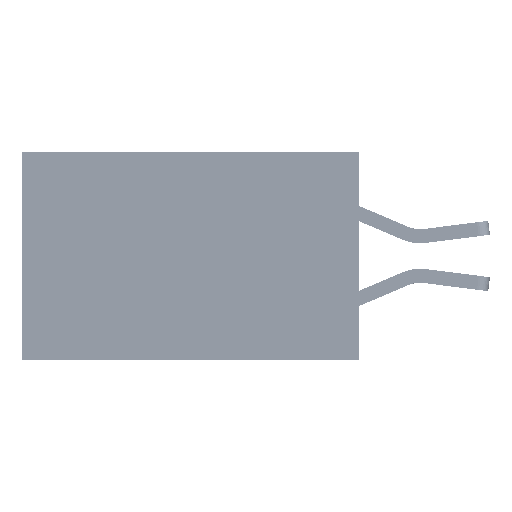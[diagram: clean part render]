
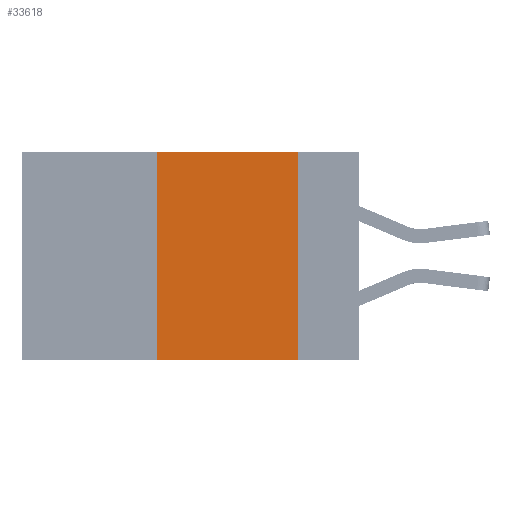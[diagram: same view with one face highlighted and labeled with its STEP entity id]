
A CAD part, left-side view. The second image highlights one B-rep face of the part: STEP entity #33618.
In plain terms, the highlighted planar face has unit normal (-1, 0, 0).
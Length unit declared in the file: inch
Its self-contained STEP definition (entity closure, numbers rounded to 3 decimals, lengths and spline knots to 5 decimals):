
#204 = LINE ( 'NONE', #19303, #33408 ) ;
#1586 = VERTEX_POINT ( 'NONE', #36401 ) ;
#2526 = VECTOR ( 'NONE', #12789, 39.37008 ) ;
#2970 = EDGE_CURVE ( 'NONE', #21396, #1586, #34443, .T. ) ;
#3030 = CARTESIAN_POINT ( 'NONE',  ( 0., 0.11, -0.37 ) ) ;
#3728 = EDGE_CURVE ( 'NONE', #21396, #26308, #35693, .T. ) ;
#4041 = ORIENTED_EDGE ( 'NONE', *, *, #3728, .T. ) ;
#4590 = LINE ( 'NONE', #7376, #32959 ) ;
#6262 = ORIENTED_EDGE ( 'NONE', *, *, #6653, .F. ) ;
#6653 = EDGE_CURVE ( 'NONE', #1586, #18485, #4590, .T. ) ;
#7141 = DIRECTION ( 'NONE',  ( 0., -1., 0. ) ) ;
#7376 = CARTESIAN_POINT ( 'NONE',  ( 0., 0.6, 0. ) ) ;
#11232 = FACE_OUTER_BOUND ( 'NONE', #19173, .T. ) ;
#11411 = PLANE ( 'NONE',  #26096 ) ;
#12393 = DIRECTION ( 'NONE',  ( 1., 0., 0. ) ) ;
#12789 = DIRECTION ( 'NONE',  ( 0., 0., 1. ) ) ;
#17364 = CARTESIAN_POINT ( 'NONE',  ( 0., 0.6, 0. ) ) ;
#17844 = DIRECTION ( 'NONE',  ( 0., 0., -1. ) ) ;
#18485 = VERTEX_POINT ( 'NONE', #23875 ) ;
#19173 = EDGE_LOOP ( 'NONE', ( #26755, #6262, #34227, #4041 ) ) ;
#19303 = CARTESIAN_POINT ( 'NONE',  ( 0., 0.11, 0. ) ) ;
#19483 = CARTESIAN_POINT ( 'NONE',  ( 0., 0.36, -0.37 ) ) ;
#21166 = CARTESIAN_POINT ( 'NONE',  ( 0., 0.6, -0.37 ) ) ;
#21396 = VERTEX_POINT ( 'NONE', #19483 ) ;
#23734 = EDGE_CURVE ( 'NONE', #18485, #26308, #204, .T. ) ;
#23875 = CARTESIAN_POINT ( 'NONE',  ( 0., 0.11, 0. ) ) ;
#26096 = AXIS2_PLACEMENT_3D ( 'NONE', #17364, #12393, #17844 ) ;
#26308 = VERTEX_POINT ( 'NONE', #3030 ) ;
#26755 = ORIENTED_EDGE ( 'NONE', *, *, #23734, .F. ) ;
#26996 = DIRECTION ( 'NONE',  ( 0., -1., 0. ) ) ;
#29404 = CARTESIAN_POINT ( 'NONE',  ( 0., 0.36, 0. ) ) ;
#32959 = VECTOR ( 'NONE', #7141, 39.37008 ) ;
#33408 = VECTOR ( 'NONE', #33503, 39.37008 ) ;
#33503 = DIRECTION ( 'NONE',  ( 0., 0., -1. ) ) ;
#33618 = ADVANCED_FACE ( 'NONE', ( #11232 ), #11411, .F. ) ;
#34227 = ORIENTED_EDGE ( 'NONE', *, *, #2970, .F. ) ;
#34443 = LINE ( 'NONE', #29404, #2526 ) ;
#34806 = VECTOR ( 'NONE', #26996, 39.37008 ) ;
#35693 = LINE ( 'NONE', #21166, #34806 ) ;
#36401 = CARTESIAN_POINT ( 'NONE',  ( 0., 0.36, 0. ) ) ;
